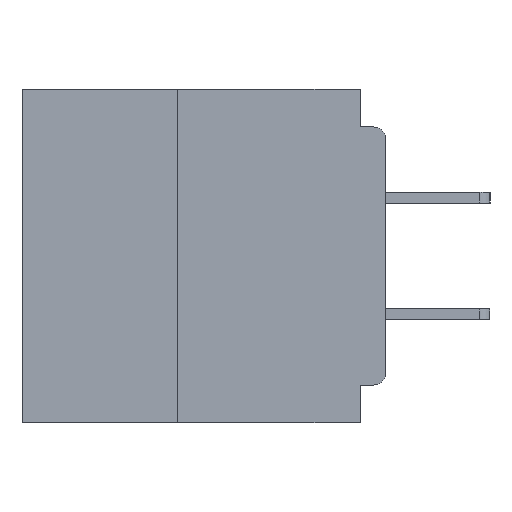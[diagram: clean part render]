
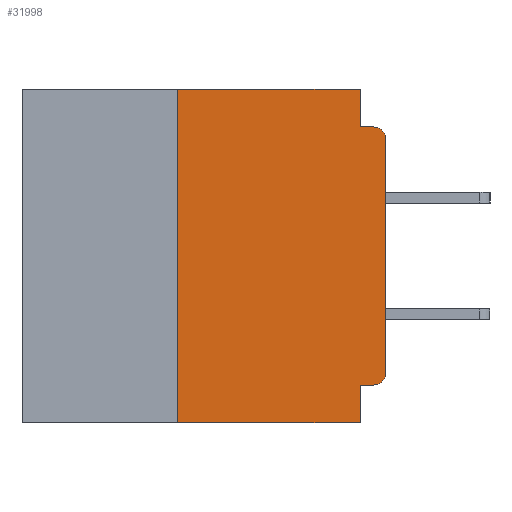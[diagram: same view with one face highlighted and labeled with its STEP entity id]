
A CAD part, left-side view. The second image highlights one B-rep face of the part: STEP entity #31998.
In plain terms, the highlighted planar face has unit normal (-1, 0, 0).
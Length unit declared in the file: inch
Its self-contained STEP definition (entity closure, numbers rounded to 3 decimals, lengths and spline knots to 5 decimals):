
#314 = CARTESIAN_POINT ( 'NONE',  ( 0., 0.031, 0. ) ) ;
#941 = VERTEX_POINT ( 'NONE', #18919 ) ;
#1797 = CARTESIAN_POINT ( 'NONE',  ( 0., 0.25, -0.4 ) ) ;
#2120 = VECTOR ( 'NONE', #35978, 39.37008 ) ;
#2345 = EDGE_CURVE ( 'NONE', #37096, #41399, #15510, .T. ) ;
#3947 = AXIS2_PLACEMENT_3D ( 'NONE', #40966, #19060, #44633 ) ;
#5940 = CARTESIAN_POINT ( 'NONE',  ( 0., 0.031, -0.045 ) ) ;
#5951 = CARTESIAN_POINT ( 'NONE',  ( 0., 0.015, -0.34 ) ) ;
#6664 = VERTEX_POINT ( 'NONE', #1797 ) ;
#6697 = ORIENTED_EDGE ( 'NONE', *, *, #29122, .F. ) ;
#7067 = VERTEX_POINT ( 'NONE', #15588 ) ;
#7416 = ORIENTED_EDGE ( 'NONE', *, *, #14288, .F. ) ;
#8157 = CIRCLE ( 'NONE', #20122, 0.015 ) ;
#9313 = LINE ( 'NONE', #45492, #37375 ) ;
#9538 = CIRCLE ( 'NONE', #26770, 0.015 ) ;
#9660 = VECTOR ( 'NONE', #44864, 39.37008 ) ;
#9706 = DIRECTION ( 'NONE',  ( 0., 0., -1. ) ) ;
#11314 = CARTESIAN_POINT ( 'NONE',  ( 0., 0.437, 0. ) ) ;
#11656 = PLANE ( 'NONE',  #3947 ) ;
#13182 = CARTESIAN_POINT ( 'NONE',  ( 0., 0.031, -0.355 ) ) ;
#13290 = EDGE_CURVE ( 'NONE', #37096, #36677, #8157, .T. ) ;
#13488 = EDGE_CURVE ( 'NONE', #6664, #7067, #17361, .T. ) ;
#13901 = CARTESIAN_POINT ( 'NONE',  ( 0., 0.031, 0. ) ) ;
#14288 = EDGE_CURVE ( 'NONE', #7067, #19973, #24193, .T. ) ;
#14481 = ORIENTED_EDGE ( 'NONE', *, *, #2345, .F. ) ;
#15510 = LINE ( 'NONE', #44020, #24090 ) ;
#15588 = CARTESIAN_POINT ( 'NONE',  ( 0., 0.25, 0. ) ) ;
#15824 = CARTESIAN_POINT ( 'NONE',  ( 0., 0.015, -0.06 ) ) ;
#16289 = FACE_OUTER_BOUND ( 'NONE', #33209, .T. ) ;
#16476 = VERTEX_POINT ( 'NONE', #5940 ) ;
#16861 = LINE ( 'NONE', #19418, #26584 ) ;
#17361 = LINE ( 'NONE', #47439, #28241 ) ;
#18540 = CARTESIAN_POINT ( 'NONE',  ( 0., 0.015, -0.045 ) ) ;
#18720 = DIRECTION ( 'NONE',  ( 0., -1., 0. ) ) ;
#18919 = CARTESIAN_POINT ( 'NONE',  ( 0., 0.031, -0.4 ) ) ;
#19060 = DIRECTION ( 'NONE',  ( 1., 0., 0. ) ) ;
#19418 = CARTESIAN_POINT ( 'NONE',  ( 0., 0., -0.045 ) ) ;
#19517 = DIRECTION ( 'NONE',  ( 0., 0., -1. ) ) ;
#19973 = VERTEX_POINT ( 'NONE', #314 ) ;
#20122 = AXIS2_PLACEMENT_3D ( 'NONE', #5951, #31652, #9706 ) ;
#21179 = VECTOR ( 'NONE', #43985, 39.37008 ) ;
#24090 = VECTOR ( 'NONE', #43046, 39.37008 ) ;
#24193 = LINE ( 'NONE', #11314, #32785 ) ;
#25270 = ORIENTED_EDGE ( 'NONE', *, *, #30461, .T. ) ;
#26158 = ORIENTED_EDGE ( 'NONE', *, *, #28218, .F. ) ;
#26584 = VECTOR ( 'NONE', #41294, 39.37008 ) ;
#26770 = AXIS2_PLACEMENT_3D ( 'NONE', #15824, #41396, #19517 ) ;
#27267 = CARTESIAN_POINT ( 'NONE',  ( 0., 0., -0.06 ) ) ;
#27282 = DIRECTION ( 'NONE',  ( 0., 0., 1. ) ) ;
#28218 = EDGE_CURVE ( 'NONE', #19973, #16476, #31545, .T. ) ;
#28241 = VECTOR ( 'NONE', #29226, 39.37008 ) ;
#29077 = CARTESIAN_POINT ( 'NONE',  ( 0., 0.015, -0.355 ) ) ;
#29122 = EDGE_CURVE ( 'NONE', #41399, #941, #37750, .T. ) ;
#29226 = DIRECTION ( 'NONE',  ( 0., 0., 1. ) ) ;
#30322 = CARTESIAN_POINT ( 'NONE',  ( 0., 0.031, -0.4 ) ) ;
#30335 = VERTEX_POINT ( 'NONE', #18540 ) ;
#30461 = EDGE_CURVE ( 'NONE', #33418, #30335, #9538, .T. ) ;
#31545 = LINE ( 'NONE', #13901, #2120 ) ;
#31652 = DIRECTION ( 'NONE',  ( -1., 0., 0. ) ) ;
#31998 = ADVANCED_FACE ( 'NONE', ( #16289 ), #11656, .F. ) ;
#32323 = ORIENTED_EDGE ( 'NONE', *, *, #13488, .F. ) ;
#32785 = VECTOR ( 'NONE', #18720, 39.37008 ) ;
#33209 = EDGE_LOOP ( 'NONE', ( #33666, #25270, #40314, #26158, #7416, #32323, #40155, #6697, #14481, #40673 ) ) ;
#33418 = VERTEX_POINT ( 'NONE', #27267 ) ;
#33666 = ORIENTED_EDGE ( 'NONE', *, *, #38456, .T. ) ;
#34270 = CARTESIAN_POINT ( 'NONE',  ( 0., 0., -0.34 ) ) ;
#35978 = DIRECTION ( 'NONE',  ( 0., 0., -1. ) ) ;
#36677 = VERTEX_POINT ( 'NONE', #34270 ) ;
#37096 = VERTEX_POINT ( 'NONE', #29077 ) ;
#37375 = VECTOR ( 'NONE', #27282, 39.37008 ) ;
#37750 = LINE ( 'NONE', #30322, #9660 ) ;
#38456 = EDGE_CURVE ( 'NONE', #36677, #33418, #9313, .T. ) ;
#40155 = ORIENTED_EDGE ( 'NONE', *, *, #43821, .T. ) ;
#40314 = ORIENTED_EDGE ( 'NONE', *, *, #41812, .F. ) ;
#40325 = CARTESIAN_POINT ( 'NONE',  ( 0., 0.437, -0.4 ) ) ;
#40673 = ORIENTED_EDGE ( 'NONE', *, *, #13290, .T. ) ;
#40966 = CARTESIAN_POINT ( 'NONE',  ( 0., 0.437, 0. ) ) ;
#41294 = DIRECTION ( 'NONE',  ( 0., -1., 0. ) ) ;
#41396 = DIRECTION ( 'NONE',  ( -1., 0., 0. ) ) ;
#41399 = VERTEX_POINT ( 'NONE', #13182 ) ;
#41812 = EDGE_CURVE ( 'NONE', #16476, #30335, #16861, .T. ) ;
#43046 = DIRECTION ( 'NONE',  ( 0., 1., 0. ) ) ;
#43821 = EDGE_CURVE ( 'NONE', #6664, #941, #46888, .T. ) ;
#43985 = DIRECTION ( 'NONE',  ( 0., -1., 0. ) ) ;
#44020 = CARTESIAN_POINT ( 'NONE',  ( 0., 0., -0.355 ) ) ;
#44633 = DIRECTION ( 'NONE',  ( 0., 0., -1. ) ) ;
#44864 = DIRECTION ( 'NONE',  ( 0., 0., -1. ) ) ;
#45492 = CARTESIAN_POINT ( 'NONE',  ( 0., 0., 0. ) ) ;
#46888 = LINE ( 'NONE', #40325, #21179 ) ;
#47439 = CARTESIAN_POINT ( 'NONE',  ( 0., 0.25, -0.4 ) ) ;
